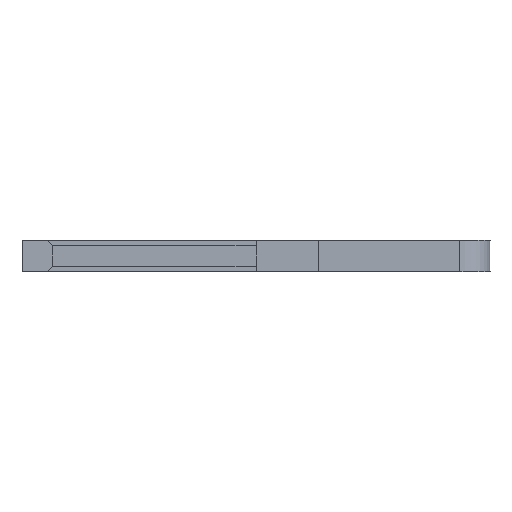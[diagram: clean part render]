
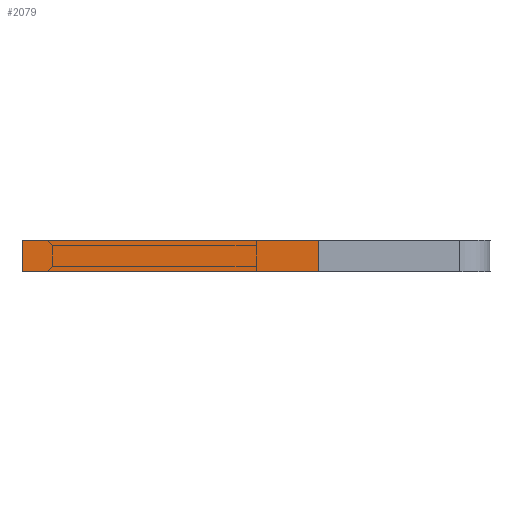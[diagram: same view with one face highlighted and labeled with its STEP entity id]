
A CAD part, left-side view. The second image highlights one B-rep face of the part: STEP entity #2079.
In plain terms, the highlighted face is planar.
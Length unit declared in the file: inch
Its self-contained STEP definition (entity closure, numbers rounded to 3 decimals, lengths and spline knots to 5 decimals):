
#6 = CARTESIAN_POINT ( 'NONE',  ( 0.01, 0.15, -0.04 ) ) ;
#139 = CARTESIAN_POINT ( 'NONE',  ( 0.01, -0.04, -0.04 ) ) ;
#165 = CARTESIAN_POINT ( 'NONE',  ( -0.01, 0.15, -0.04 ) ) ;
#170 = ORIENTED_EDGE ( 'NONE', *, *, #238, .F. ) ;
#238 = EDGE_CURVE ( 'NONE', #968, #1208, #790, .T. ) ;
#310 = CARTESIAN_POINT ( 'NONE',  ( 0.01, -0.04, -0.04 ) ) ;
#399 = LINE ( 'NONE', #2128, #2186 ) ;
#656 = CARTESIAN_POINT ( 'NONE',  ( 0.01, 0.15, -0.04 ) ) ;
#682 = DIRECTION ( 'NONE',  ( 0., 1., 0. ) ) ;
#790 = LINE ( 'NONE', #656, #1824 ) ;
#848 = FACE_OUTER_BOUND ( 'NONE', #1125, .T. ) ;
#865 = CARTESIAN_POINT ( 'NONE',  ( -0.01, 0.15, -0.04 ) ) ;
#884 = PLANE ( 'NONE',  #1141 ) ;
#968 = VERTEX_POINT ( 'NONE', #139 ) ;
#975 = EDGE_CURVE ( 'NONE', #2120, #1089, #1607, .T. ) ;
#1049 = ORIENTED_EDGE ( 'NONE', *, *, #1847, .T. ) ;
#1089 = VERTEX_POINT ( 'NONE', #165 ) ;
#1125 = EDGE_LOOP ( 'NONE', ( #1694, #1468, #170, #1049 ) ) ;
#1141 = AXIS2_PLACEMENT_3D ( 'NONE', #1422, #1402, #1570 ) ;
#1201 = DIRECTION ( 'NONE',  ( 0., 1., 0. ) ) ;
#1208 = VERTEX_POINT ( 'NONE', #6 ) ;
#1402 = DIRECTION ( 'NONE',  ( 0., 0., 1. ) ) ;
#1422 = CARTESIAN_POINT ( 'NONE',  ( 0.01, 0.15, -0.04 ) ) ;
#1468 = ORIENTED_EDGE ( 'NONE', *, *, #1979, .F. ) ;
#1537 = VECTOR ( 'NONE', #1768, 39.37008 ) ;
#1570 = DIRECTION ( 'NONE',  ( 1., 0., 0. ) ) ;
#1591 = DIRECTION ( 'NONE',  ( -1., 0., 0. ) ) ;
#1607 = LINE ( 'NONE', #865, #2017 ) ;
#1694 = ORIENTED_EDGE ( 'NONE', *, *, #975, .T. ) ;
#1728 = LINE ( 'NONE', #310, #1537 ) ;
#1768 = DIRECTION ( 'NONE',  ( -1., 0., 0. ) ) ;
#1824 = VECTOR ( 'NONE', #1201, 39.37008 ) ;
#1847 = EDGE_CURVE ( 'NONE', #968, #2120, #1728, .T. ) ;
#1979 = EDGE_CURVE ( 'NONE', #1208, #1089, #399, .T. ) ;
#2017 = VECTOR ( 'NONE', #682, 39.37008 ) ;
#2079 = ADVANCED_FACE ( 'NONE', ( #848 ), #884, .F. ) ;
#2102 = CARTESIAN_POINT ( 'NONE',  ( -0.01, -0.04, -0.04 ) ) ;
#2120 = VERTEX_POINT ( 'NONE', #2102 ) ;
#2128 = CARTESIAN_POINT ( 'NONE',  ( 0.01, 0.15, -0.04 ) ) ;
#2186 = VECTOR ( 'NONE', #1591, 39.37008 ) ;
